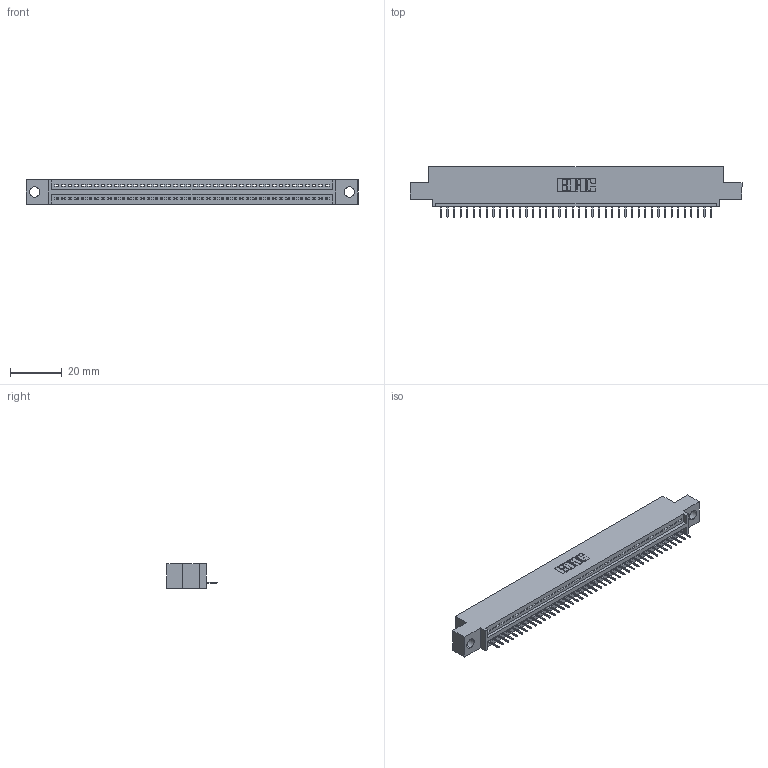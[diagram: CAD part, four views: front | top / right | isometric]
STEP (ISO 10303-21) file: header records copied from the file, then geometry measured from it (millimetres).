
FILE_DESCRIPTION (( 'STEP AP203' ), '1' );
FILE_NAME ('345-042-524-404.STEP', '2021-05-26T15:02:11', ( '' ), ( '' ), 'SwSTEP 2.0', 'SolidWorks 2020', '' );
FILE_SCHEMA (( 'CONFIG_CONTROL_DESIGN' ));
Length unit declared in the file: inch
Products named in the file (3): 345-042-524-404; 345-292-001_345-293-124; 345 Part_0.110 Offset - 0.156 Dia-TI
Assembly tree (43 placements, depth 2):
  345-042-524-404
    345 Part_0.110 Offset - 0.156 Dia-TI
    345-292-001_345-293-124  x42
Bounding box: 127.89 x 19.35 x 9.4 mm (x, y, z)
Volume: 11801.8 mm3; surface area: 15077.4 mm2
Topology: 43 solids, 43 shells, 2748 faces, 7949 edges, 5130 vertices
Faces by surface type: plane 2030, cylinder 718
Entity records: 32235 total; most frequent: CARTESIAN_POINT 5592, ORIENTED_EDGE 5566, DIRECTION 4883, EDGE_CURVE 2783, VECTOR 2487, LINE 2487, VERTEX_POINT 1850, AXIS2_PLACEMENT_3D 1198
